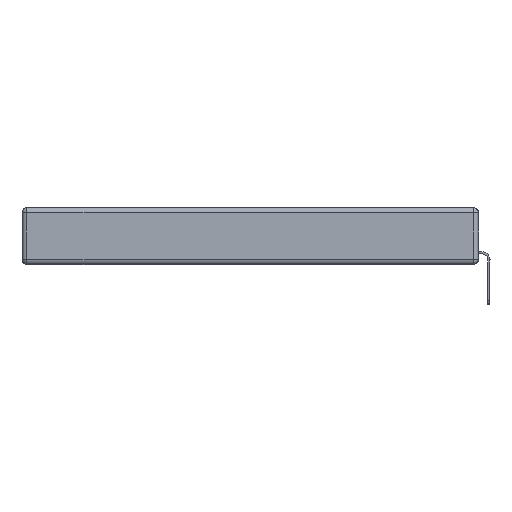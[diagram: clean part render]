
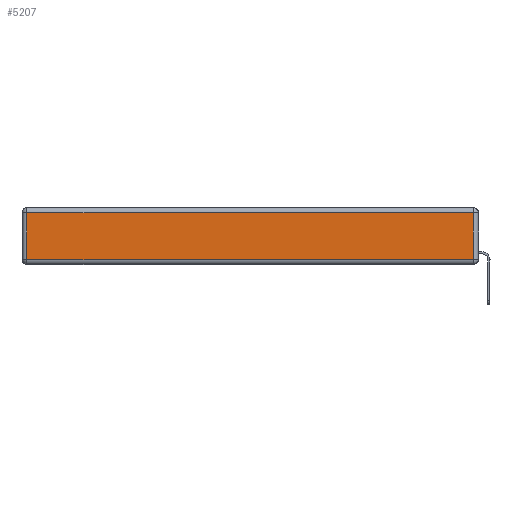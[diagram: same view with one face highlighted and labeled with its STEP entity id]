
A CAD part, left-side view. The second image highlights one B-rep face of the part: STEP entity #5207.
In plain terms, the highlighted planar face has unit normal (-1, 0, 0).
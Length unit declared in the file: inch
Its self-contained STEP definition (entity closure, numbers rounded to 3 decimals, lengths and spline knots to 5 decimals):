
#180 = CARTESIAN_POINT ( 'NONE',  ( 0., 2.72, -0.313 ) ) ;
#905 = DIRECTION ( 'NONE',  ( -1., 0., 0. ) ) ;
#1100 = CARTESIAN_POINT ( 'NONE',  ( 0., 2.75, -0.03 ) ) ;
#2150 = VERTEX_POINT ( 'NONE', #180 ) ;
#3417 = CARTESIAN_POINT ( 'NONE',  ( 0., 0., -0.343 ) ) ;
#3771 = DIRECTION ( 'NONE',  ( 0., -1., 0. ) ) ;
#4609 = EDGE_CURVE ( 'NONE', #13312, #12223, #8525, .T. ) ;
#4754 = CARTESIAN_POINT ( 'NONE',  ( 0., 2.72, -0.343 ) ) ;
#5024 = LINE ( 'NONE', #5225, #18047 ) ;
#5207 = ADVANCED_FACE ( 'NONE', ( #12076 ), #17978, .T. ) ;
#5225 = CARTESIAN_POINT ( 'NONE',  ( 0., 0., -0.313 ) ) ;
#6210 = ORIENTED_EDGE ( 'NONE', *, *, #16178, .T. ) ;
#7216 = LINE ( 'NONE', #11727, #11591 ) ;
#8027 = AXIS2_PLACEMENT_3D ( 'NONE', #3417, #905, #18543 ) ;
#8048 = VERTEX_POINT ( 'NONE', #9574 ) ;
#8525 = LINE ( 'NONE', #1100, #18184 ) ;
#9574 = CARTESIAN_POINT ( 'NONE',  ( 0., 0.03, -0.313 ) ) ;
#10292 = ORIENTED_EDGE ( 'NONE', *, *, #17286, .T. ) ;
#11591 = VECTOR ( 'NONE', #18797, 39.37008 ) ;
#11727 = CARTESIAN_POINT ( 'NONE',  ( 0., 0.03, -0.343 ) ) ;
#12052 = EDGE_CURVE ( 'NONE', #12223, #2150, #17963, .T. ) ;
#12076 = FACE_OUTER_BOUND ( 'NONE', #14642, .T. ) ;
#12223 = VERTEX_POINT ( 'NONE', #18441 ) ;
#12709 = VECTOR ( 'NONE', #14779, 39.37008 ) ;
#13312 = VERTEX_POINT ( 'NONE', #13379 ) ;
#13379 = CARTESIAN_POINT ( 'NONE',  ( 0., 0.03, -0.03 ) ) ;
#14408 = DIRECTION ( 'NONE',  ( 0., 1., 0. ) ) ;
#14642 = EDGE_LOOP ( 'NONE', ( #10292, #6210, #17177, #14667 ) ) ;
#14667 = ORIENTED_EDGE ( 'NONE', *, *, #12052, .T. ) ;
#14779 = DIRECTION ( 'NONE',  ( 0., 0., -1. ) ) ;
#16178 = EDGE_CURVE ( 'NONE', #8048, #13312, #7216, .T. ) ;
#17177 = ORIENTED_EDGE ( 'NONE', *, *, #4609, .T. ) ;
#17286 = EDGE_CURVE ( 'NONE', #2150, #8048, #5024, .T. ) ;
#17963 = LINE ( 'NONE', #4754, #12709 ) ;
#17978 = PLANE ( 'NONE',  #8027 ) ;
#18047 = VECTOR ( 'NONE', #3771, 39.37008 ) ;
#18184 = VECTOR ( 'NONE', #14408, 39.37008 ) ;
#18441 = CARTESIAN_POINT ( 'NONE',  ( 0., 2.72, -0.03 ) ) ;
#18543 = DIRECTION ( 'NONE',  ( 0., 0., 1. ) ) ;
#18797 = DIRECTION ( 'NONE',  ( 0., 0., 1. ) ) ;
